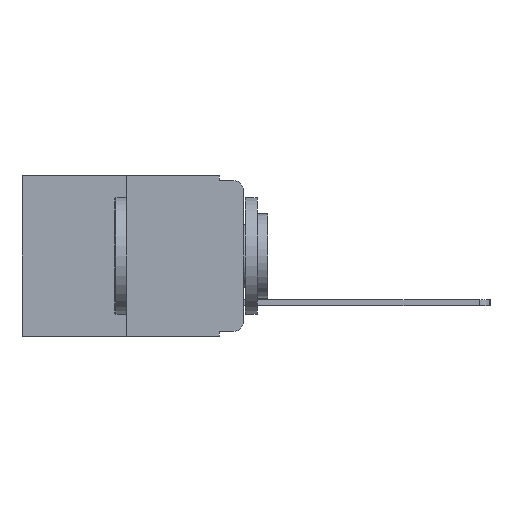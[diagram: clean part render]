
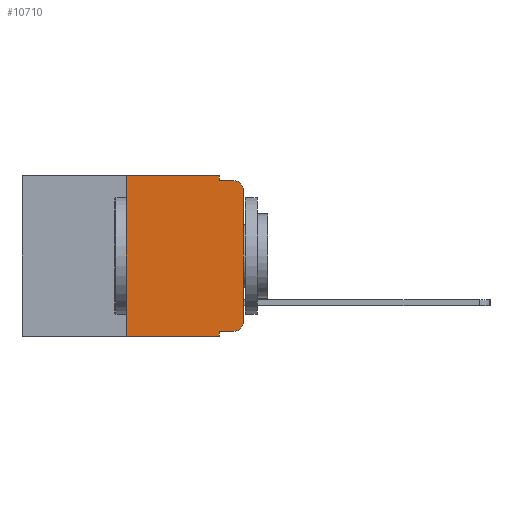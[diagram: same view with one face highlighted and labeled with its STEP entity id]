
A CAD part, left-side view. The second image highlights one B-rep face of the part: STEP entity #10710.
In plain terms, the highlighted planar face has unit normal (-1, 0, 0).
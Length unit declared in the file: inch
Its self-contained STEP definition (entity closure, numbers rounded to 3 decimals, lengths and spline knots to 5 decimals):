
#76 = ORIENTED_EDGE ( 'NONE', *, *, #15722, .F. ) ;
#141 = DIRECTION ( 'NONE',  ( 0., -1., 0. ) ) ;
#149 = VECTOR ( 'NONE', #3171, 39.37008 ) ;
#214 = CIRCLE ( 'NONE', #13348, 0.02 ) ;
#464 = VERTEX_POINT ( 'NONE', #5344 ) ;
#803 = DIRECTION ( 'NONE',  ( 0., 0., -1. ) ) ;
#991 = ORIENTED_EDGE ( 'NONE', *, *, #3787, .T. ) ;
#1021 = CARTESIAN_POINT ( 'NONE',  ( 0., 0.051, 0. ) ) ;
#1251 = EDGE_CURVE ( 'NONE', #464, #10195, #2001, .T. ) ;
#1769 = VECTOR ( 'NONE', #16143, 39.37008 ) ;
#1800 = CARTESIAN_POINT ( 'NONE',  ( 0., 0.473, 0. ) ) ;
#1903 = CARTESIAN_POINT ( 'NONE',  ( 0., 0.25, 0. ) ) ;
#1930 = EDGE_CURVE ( 'NONE', #2288, #3252, #12366, .T. ) ;
#1938 = VERTEX_POINT ( 'NONE', #14204 ) ;
#2001 = LINE ( 'NONE', #1903, #12189 ) ;
#2288 = VERTEX_POINT ( 'NONE', #16701 ) ;
#2306 = EDGE_CURVE ( 'NONE', #11100, #2288, #214, .T. ) ;
#2613 = FACE_OUTER_BOUND ( 'NONE', #4821, .T. ) ;
#3171 = DIRECTION ( 'NONE',  ( 0., -1., 0. ) ) ;
#3207 = VECTOR ( 'NONE', #141, 39.37008 ) ;
#3252 = VERTEX_POINT ( 'NONE', #4429 ) ;
#3430 = EDGE_CURVE ( 'NONE', #16691, #1938, #4483, .T. ) ;
#3483 = PLANE ( 'NONE',  #5656 ) ;
#3498 = CARTESIAN_POINT ( 'NONE',  ( 0., 0.25, 0. ) ) ;
#3563 = LINE ( 'NONE', #16545, #7114 ) ;
#3787 = EDGE_CURVE ( 'NONE', #6909, #11100, #15258, .T. ) ;
#4030 = CARTESIAN_POINT ( 'NONE',  ( 0., 0.051, -0.333 ) ) ;
#4429 = CARTESIAN_POINT ( 'NONE',  ( 0., 0., -0.03 ) ) ;
#4483 = LINE ( 'NONE', #5373, #3207 ) ;
#4710 = CARTESIAN_POINT ( 'NONE',  ( 0., 0.051, -0.343 ) ) ;
#4821 = EDGE_LOOP ( 'NONE', ( #9957, #16773, #6891, #13818, #76, #7312, #14228, #7717, #991, #5003 ) ) ;
#4866 = VECTOR ( 'NONE', #13820, 39.37008 ) ;
#5003 = ORIENTED_EDGE ( 'NONE', *, *, #2306, .T. ) ;
#5344 = CARTESIAN_POINT ( 'NONE',  ( 0., 0.25, -0.343 ) ) ;
#5373 = CARTESIAN_POINT ( 'NONE',  ( 0., 0.051, -0.01 ) ) ;
#5545 = DIRECTION ( 'NONE',  ( 0., 0., 1. ) ) ;
#5656 = AXIS2_PLACEMENT_3D ( 'NONE', #12710, #13991, #6165 ) ;
#6165 = DIRECTION ( 'NONE',  ( 0., 0., -1. ) ) ;
#6480 = LINE ( 'NONE', #6779, #13024 ) ;
#6779 = CARTESIAN_POINT ( 'NONE',  ( 0., 0.051, 0. ) ) ;
#6891 = ORIENTED_EDGE ( 'NONE', *, *, #3430, .F. ) ;
#6909 = VERTEX_POINT ( 'NONE', #4030 ) ;
#7014 = CARTESIAN_POINT ( 'NONE',  ( 0., 0.051, -0.01 ) ) ;
#7114 = VECTOR ( 'NONE', #10154, 39.37008 ) ;
#7312 = ORIENTED_EDGE ( 'NONE', *, *, #1251, .F. ) ;
#7378 = LINE ( 'NONE', #1800, #149 ) ;
#7709 = CIRCLE ( 'NONE', #12887, 0.02 ) ;
#7717 = ORIENTED_EDGE ( 'NONE', *, *, #8732, .F. ) ;
#8440 = EDGE_CURVE ( 'NONE', #464, #10664, #3563, .T. ) ;
#8576 = CARTESIAN_POINT ( 'NONE',  ( 0., 0.02, -0.313 ) ) ;
#8732 = EDGE_CURVE ( 'NONE', #6909, #10664, #6480, .T. ) ;
#8799 = DIRECTION ( 'NONE',  ( -1., 0., 0. ) ) ;
#9049 = EDGE_CURVE ( 'NONE', #3252, #1938, #7709, .T. ) ;
#9372 = VECTOR ( 'NONE', #14251, 39.37008 ) ;
#9957 = ORIENTED_EDGE ( 'NONE', *, *, #1930, .T. ) ;
#10115 = CARTESIAN_POINT ( 'NONE',  ( 0., 0., 0. ) ) ;
#10154 = DIRECTION ( 'NONE',  ( 0., -1., 0. ) ) ;
#10195 = VERTEX_POINT ( 'NONE', #3498 ) ;
#10664 = VERTEX_POINT ( 'NONE', #4710 ) ;
#10710 = ADVANCED_FACE ( 'NONE', ( #2613 ), #3483, .F. ) ;
#11100 = VERTEX_POINT ( 'NONE', #13523 ) ;
#11550 = VERTEX_POINT ( 'NONE', #16883 ) ;
#12189 = VECTOR ( 'NONE', #5545, 39.37008 ) ;
#12366 = LINE ( 'NONE', #10115, #1769 ) ;
#12710 = CARTESIAN_POINT ( 'NONE',  ( 0., 0.473, 0. ) ) ;
#12887 = AXIS2_PLACEMENT_3D ( 'NONE', #16526, #8799, #803 ) ;
#13024 = VECTOR ( 'NONE', #13328, 39.37008 ) ;
#13265 = LINE ( 'NONE', #1021, #9372 ) ;
#13316 = CARTESIAN_POINT ( 'NONE',  ( 0., 0.051, -0.333 ) ) ;
#13328 = DIRECTION ( 'NONE',  ( 0., 0., -1. ) ) ;
#13348 = AXIS2_PLACEMENT_3D ( 'NONE', #8576, #16230, #16465 ) ;
#13523 = CARTESIAN_POINT ( 'NONE',  ( 0., 0.02, -0.333 ) ) ;
#13818 = ORIENTED_EDGE ( 'NONE', *, *, #15969, .F. ) ;
#13820 = DIRECTION ( 'NONE',  ( 0., -1., 0. ) ) ;
#13991 = DIRECTION ( 'NONE',  ( 1., 0., 0. ) ) ;
#14204 = CARTESIAN_POINT ( 'NONE',  ( 0., 0.02, -0.01 ) ) ;
#14228 = ORIENTED_EDGE ( 'NONE', *, *, #8440, .T. ) ;
#14251 = DIRECTION ( 'NONE',  ( 0., 0., -1. ) ) ;
#15258 = LINE ( 'NONE', #13316, #4866 ) ;
#15722 = EDGE_CURVE ( 'NONE', #10195, #11550, #7378, .T. ) ;
#15969 = EDGE_CURVE ( 'NONE', #11550, #16691, #13265, .T. ) ;
#16143 = DIRECTION ( 'NONE',  ( 0., 0., 1. ) ) ;
#16230 = DIRECTION ( 'NONE',  ( -1., 0., 0. ) ) ;
#16465 = DIRECTION ( 'NONE',  ( 0., 0., -1. ) ) ;
#16526 = CARTESIAN_POINT ( 'NONE',  ( 0., 0.02, -0.03 ) ) ;
#16545 = CARTESIAN_POINT ( 'NONE',  ( 0., 0.473, -0.343 ) ) ;
#16691 = VERTEX_POINT ( 'NONE', #7014 ) ;
#16701 = CARTESIAN_POINT ( 'NONE',  ( 0., 0., -0.313 ) ) ;
#16773 = ORIENTED_EDGE ( 'NONE', *, *, #9049, .T. ) ;
#16883 = CARTESIAN_POINT ( 'NONE',  ( 0., 0.051, 0. ) ) ;
